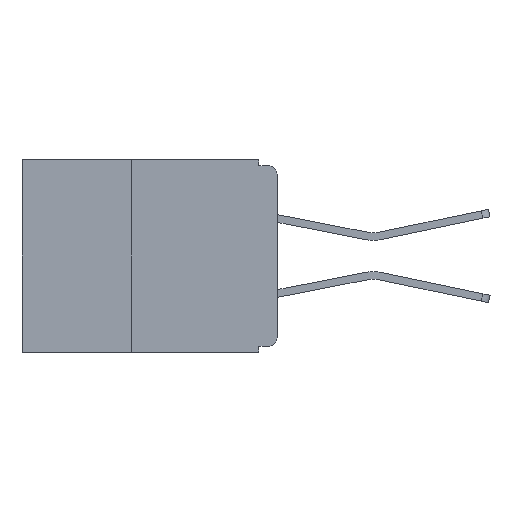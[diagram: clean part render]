
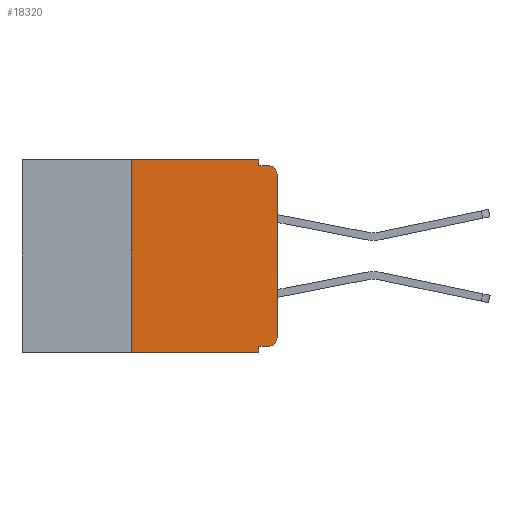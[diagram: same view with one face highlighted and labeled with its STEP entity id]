
A CAD part, left-side view. The second image highlights one B-rep face of the part: STEP entity #18320.
In plain terms, the highlighted planar face has unit normal (-1, 0, 0).
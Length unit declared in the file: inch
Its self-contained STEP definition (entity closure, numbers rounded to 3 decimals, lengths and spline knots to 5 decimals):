
#54 = CARTESIAN_POINT ( 'NONE',  ( 0., 0., 0. ) ) ;
#172 = DIRECTION ( 'NONE',  ( 0., 0., 1. ) ) ;
#269 = CARTESIAN_POINT ( 'NONE',  ( 0., 0.015, -0.025 ) ) ;
#409 = CARTESIAN_POINT ( 'NONE',  ( 0., 0.25, -0.33 ) ) ;
#418 = LINE ( 'NONE', #18024, #12294 ) ;
#492 = EDGE_CURVE ( 'NONE', #8478, #12596, #12739, .T. ) ;
#960 = EDGE_CURVE ( 'NONE', #11968, #9706, #418, .T. ) ;
#1186 = DIRECTION ( 'NONE',  ( 0., 0., -1. ) ) ;
#1204 = EDGE_CURVE ( 'NONE', #5988, #9706, #8193, .T. ) ;
#1267 = DIRECTION ( 'NONE',  ( -1., 0., 0. ) ) ;
#2061 = EDGE_CURVE ( 'NONE', #11887, #13250, #10434, .T. ) ;
#2332 = AXIS2_PLACEMENT_3D ( 'NONE', #18937, #4345, #14619 ) ;
#2510 = ORIENTED_EDGE ( 'NONE', *, *, #6376, .T. ) ;
#2763 = CARTESIAN_POINT ( 'NONE',  ( 0., 0.031, -0.01 ) ) ;
#2833 = PLANE ( 'NONE',  #2332 ) ;
#2905 = CARTESIAN_POINT ( 'NONE',  ( 0., 0.031, 0. ) ) ;
#3343 = VERTEX_POINT ( 'NONE', #7780 ) ;
#3393 = CARTESIAN_POINT ( 'NONE',  ( 0., 0.25, 0. ) ) ;
#3565 = CARTESIAN_POINT ( 'NONE',  ( 0., 0.015, -0.305 ) ) ;
#4345 = DIRECTION ( 'NONE',  ( 1., 0., 0. ) ) ;
#4503 = DIRECTION ( 'NONE',  ( 0., 1., 0. ) ) ;
#4522 = VECTOR ( 'NONE', #172, 39.37008 ) ;
#4742 = LINE ( 'NONE', #13282, #12132 ) ;
#5089 = DIRECTION ( 'NONE',  ( 0., 0., -1. ) ) ;
#5459 = EDGE_CURVE ( 'NONE', #11887, #8478, #16234, .T. ) ;
#5571 = CARTESIAN_POINT ( 'NONE',  ( 0., 0.437, 0. ) ) ;
#5658 = EDGE_CURVE ( 'NONE', #8046, #9133, #4742, .T. ) ;
#5988 = VERTEX_POINT ( 'NONE', #6729 ) ;
#6042 = VECTOR ( 'NONE', #17297, 39.37008 ) ;
#6257 = ORIENTED_EDGE ( 'NONE', *, *, #5459, .F. ) ;
#6376 = EDGE_CURVE ( 'NONE', #3343, #5988, #14044, .T. ) ;
#6399 = CARTESIAN_POINT ( 'NONE',  ( 0., 0.031, -0.32 ) ) ;
#6549 = FACE_OUTER_BOUND ( 'NONE', #15014, .T. ) ;
#6729 = CARTESIAN_POINT ( 'NONE',  ( 0., 0., -0.025 ) ) ;
#6759 = VECTOR ( 'NONE', #10508, 39.37008 ) ;
#6795 = ORIENTED_EDGE ( 'NONE', *, *, #2061, .T. ) ;
#7165 = CARTESIAN_POINT ( 'NONE',  ( 0., 0.015, -0.32 ) ) ;
#7322 = CARTESIAN_POINT ( 'NONE',  ( 0., 0.031, -0.33 ) ) ;
#7780 = CARTESIAN_POINT ( 'NONE',  ( 0., 0., -0.305 ) ) ;
#8046 = VERTEX_POINT ( 'NONE', #7165 ) ;
#8193 = CIRCLE ( 'NONE', #11826, 0.015 ) ;
#8478 = VERTEX_POINT ( 'NONE', #3393 ) ;
#9115 = AXIS2_PLACEMENT_3D ( 'NONE', #3565, #13862, #5089 ) ;
#9133 = VERTEX_POINT ( 'NONE', #6399 ) ;
#9357 = ORIENTED_EDGE ( 'NONE', *, *, #10302, .F. ) ;
#9706 = VERTEX_POINT ( 'NONE', #12283 ) ;
#10302 = EDGE_CURVE ( 'NONE', #9133, #13250, #15027, .T. ) ;
#10434 = LINE ( 'NONE', #11424, #6042 ) ;
#10508 = DIRECTION ( 'NONE',  ( 0., 0., 1. ) ) ;
#10892 = ORIENTED_EDGE ( 'NONE', *, *, #1204, .T. ) ;
#11424 = CARTESIAN_POINT ( 'NONE',  ( 0., 0.437, -0.33 ) ) ;
#11826 = AXIS2_PLACEMENT_3D ( 'NONE', #269, #1267, #1186 ) ;
#11887 = VERTEX_POINT ( 'NONE', #17300 ) ;
#11968 = VERTEX_POINT ( 'NONE', #2763 ) ;
#12132 = VECTOR ( 'NONE', #4503, 39.37008 ) ;
#12178 = LINE ( 'NONE', #2905, #18507 ) ;
#12283 = CARTESIAN_POINT ( 'NONE',  ( 0., 0.015, -0.01 ) ) ;
#12294 = VECTOR ( 'NONE', #14856, 39.37008 ) ;
#12564 = ORIENTED_EDGE ( 'NONE', *, *, #5658, .F. ) ;
#12596 = VERTEX_POINT ( 'NONE', #17447 ) ;
#12739 = LINE ( 'NONE', #5571, #17085 ) ;
#13250 = VERTEX_POINT ( 'NONE', #7322 ) ;
#13282 = CARTESIAN_POINT ( 'NONE',  ( 0., 0., -0.32 ) ) ;
#13623 = DIRECTION ( 'NONE',  ( 0., 0., -1. ) ) ;
#13862 = DIRECTION ( 'NONE',  ( -1., 0., 0. ) ) ;
#14044 = LINE ( 'NONE', #54, #6759 ) ;
#14247 = ORIENTED_EDGE ( 'NONE', *, *, #14273, .F. ) ;
#14273 = EDGE_CURVE ( 'NONE', #12596, #11968, #12178, .T. ) ;
#14382 = DIRECTION ( 'NONE',  ( 0., -1., 0. ) ) ;
#14562 = VECTOR ( 'NONE', #13623, 39.37008 ) ;
#14619 = DIRECTION ( 'NONE',  ( 0., 0., -1. ) ) ;
#14684 = DIRECTION ( 'NONE',  ( 0., 0., -1. ) ) ;
#14856 = DIRECTION ( 'NONE',  ( 0., -1., 0. ) ) ;
#15014 = EDGE_LOOP ( 'NONE', ( #2510, #10892, #18786, #14247, #16093, #6257, #6795, #9357, #12564, #18928 ) ) ;
#15027 = LINE ( 'NONE', #16507, #14562 ) ;
#16093 = ORIENTED_EDGE ( 'NONE', *, *, #492, .F. ) ;
#16234 = LINE ( 'NONE', #409, #4522 ) ;
#16379 = CIRCLE ( 'NONE', #9115, 0.015 ) ;
#16507 = CARTESIAN_POINT ( 'NONE',  ( 0., 0.031, -0.33 ) ) ;
#17085 = VECTOR ( 'NONE', #14382, 39.37008 ) ;
#17297 = DIRECTION ( 'NONE',  ( 0., -1., 0. ) ) ;
#17300 = CARTESIAN_POINT ( 'NONE',  ( 0., 0.25, -0.33 ) ) ;
#17447 = CARTESIAN_POINT ( 'NONE',  ( 0., 0.031, 0. ) ) ;
#18012 = EDGE_CURVE ( 'NONE', #8046, #3343, #16379, .T. ) ;
#18024 = CARTESIAN_POINT ( 'NONE',  ( 0., 0., -0.01 ) ) ;
#18320 = ADVANCED_FACE ( 'NONE', ( #6549 ), #2833, .F. ) ;
#18507 = VECTOR ( 'NONE', #14684, 39.37008 ) ;
#18786 = ORIENTED_EDGE ( 'NONE', *, *, #960, .F. ) ;
#18928 = ORIENTED_EDGE ( 'NONE', *, *, #18012, .T. ) ;
#18937 = CARTESIAN_POINT ( 'NONE',  ( 0., 0.437, 0. ) ) ;
